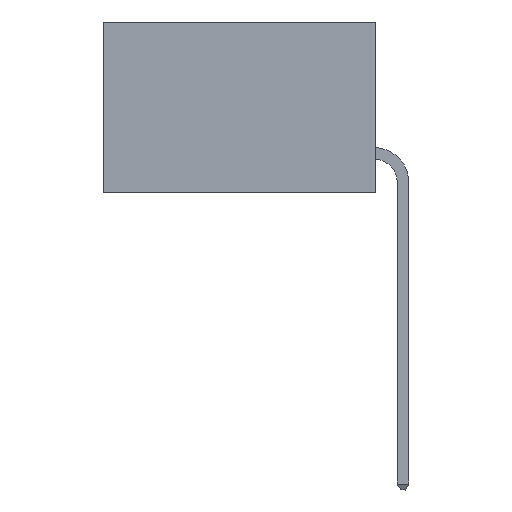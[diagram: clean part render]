
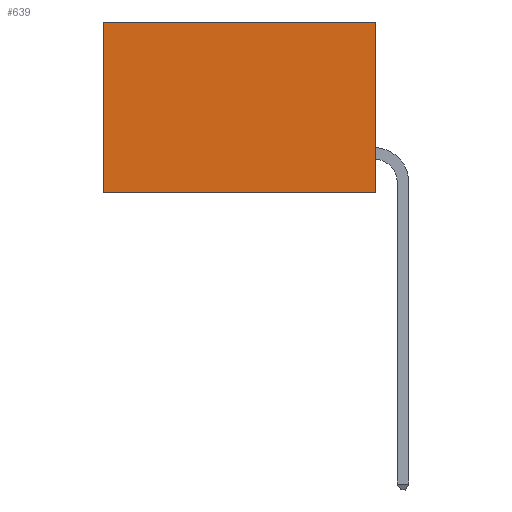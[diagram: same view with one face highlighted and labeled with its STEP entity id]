
A CAD part, left-side view. The second image highlights one B-rep face of the part: STEP entity #639.
In plain terms, the highlighted planar face has unit normal (-1, 0, 0).
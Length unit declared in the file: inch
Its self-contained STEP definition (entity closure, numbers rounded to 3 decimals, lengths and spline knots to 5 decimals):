
#25 = CARTESIAN_POINT ( 'NONE',  ( 0.277, 0.59, -0.37 ) ) ;
#27 = VERTEX_POINT ( 'NONE', #25 ) ;
#255 = CARTESIAN_POINT ( 'NONE',  ( 0.277, 0., -0.37 ) ) ;
#527 = CARTESIAN_POINT ( 'NONE',  ( 0.277, 0., -0.37 ) ) ;
#623 = EDGE_LOOP ( 'NONE', ( #5546, #7234, #8801, #2011 ) ) ;
#639 = ADVANCED_FACE ( 'NONE', ( #4499 ), #3712, .F. ) ;
#1142 = DIRECTION ( 'NONE',  ( 0., 0., -1. ) ) ;
#1232 = DIRECTION ( 'NONE',  ( 0., 1., 0. ) ) ;
#1610 = VECTOR ( 'NONE', #1232, 39.37008 ) ;
#1709 = CARTESIAN_POINT ( 'NONE',  ( 0.277, 0., 0. ) ) ;
#2011 = ORIENTED_EDGE ( 'NONE', *, *, #6549, .T. ) ;
#2034 = EDGE_CURVE ( 'NONE', #5455, #27, #8651, .T. ) ;
#2216 = LINE ( 'NONE', #5288, #8942 ) ;
#2235 = DIRECTION ( 'NONE',  ( 0., 0., -1. ) ) ;
#2806 = CARTESIAN_POINT ( 'NONE',  ( 0.277, 0., 0. ) ) ;
#3626 = AXIS2_PLACEMENT_3D ( 'NONE', #5299, #8414, #2235 ) ;
#3712 = PLANE ( 'NONE',  #3626 ) ;
#4050 = CARTESIAN_POINT ( 'NONE',  ( 0.277, 0.59, 0. ) ) ;
#4385 = VERTEX_POINT ( 'NONE', #527 ) ;
#4499 = FACE_OUTER_BOUND ( 'NONE', #623, .T. ) ;
#4523 = VERTEX_POINT ( 'NONE', #1709 ) ;
#4700 = CARTESIAN_POINT ( 'NONE',  ( 0.277, 0.59, -0.37 ) ) ;
#4718 = DIRECTION ( 'NONE',  ( 0., 0., -1. ) ) ;
#5180 = EDGE_CURVE ( 'NONE', #4385, #27, #2216, .T. ) ;
#5288 = CARTESIAN_POINT ( 'NONE',  ( 0.277, 0., -0.37 ) ) ;
#5299 = CARTESIAN_POINT ( 'NONE',  ( 0.277, 0., -0.37 ) ) ;
#5455 = VERTEX_POINT ( 'NONE', #4050 ) ;
#5546 = ORIENTED_EDGE ( 'NONE', *, *, #2034, .T. ) ;
#5937 = DIRECTION ( 'NONE',  ( 0., 1., 0. ) ) ;
#6151 = LINE ( 'NONE', #255, #6358 ) ;
#6358 = VECTOR ( 'NONE', #1142, 39.37008 ) ;
#6549 = EDGE_CURVE ( 'NONE', #4523, #5455, #8549, .T. ) ;
#7234 = ORIENTED_EDGE ( 'NONE', *, *, #5180, .F. ) ;
#7469 = EDGE_CURVE ( 'NONE', #4523, #4385, #6151, .T. ) ;
#8288 = VECTOR ( 'NONE', #4718, 39.37008 ) ;
#8414 = DIRECTION ( 'NONE',  ( 1., 0., 0. ) ) ;
#8549 = LINE ( 'NONE', #2806, #1610 ) ;
#8651 = LINE ( 'NONE', #4700, #8288 ) ;
#8801 = ORIENTED_EDGE ( 'NONE', *, *, #7469, .F. ) ;
#8942 = VECTOR ( 'NONE', #5937, 39.37008 ) ;
